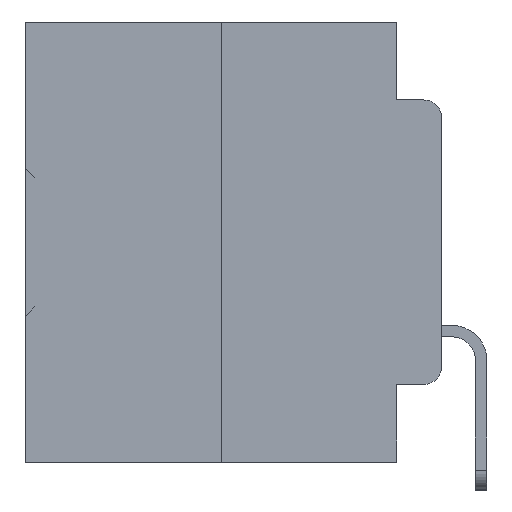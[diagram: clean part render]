
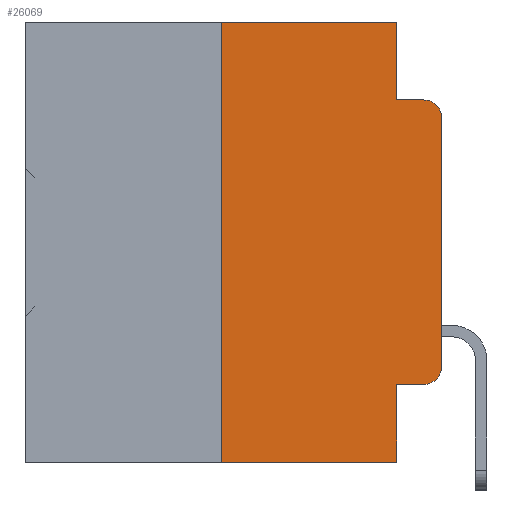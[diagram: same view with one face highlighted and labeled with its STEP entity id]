
A CAD part, left-side view. The second image highlights one B-rep face of the part: STEP entity #26069.
In plain terms, the highlighted planar face has unit normal (-1, 0, 0).
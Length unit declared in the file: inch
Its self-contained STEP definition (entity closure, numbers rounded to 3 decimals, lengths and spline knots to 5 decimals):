
#166 = LINE ( 'NONE', #28199, #23881 ) ;
#250 = VECTOR ( 'NONE', #28314, 39.37008 ) ;
#1336 = DIRECTION ( 'NONE',  ( -1., 0., 0. ) ) ;
#1528 = VERTEX_POINT ( 'NONE', #11129 ) ;
#2010 = VERTEX_POINT ( 'NONE', #10400 ) ;
#2981 = EDGE_CURVE ( 'NONE', #5622, #13626, #22046, .T. ) ;
#3457 = ORIENTED_EDGE ( 'NONE', *, *, #6452, .T. ) ;
#3941 = LINE ( 'NONE', #6048, #19441 ) ;
#4427 = CARTESIAN_POINT ( 'NONE',  ( 0., 0.473, 0. ) ) ;
#5622 = VERTEX_POINT ( 'NONE', #19685 ) ;
#5804 = DIRECTION ( 'NONE',  ( 0., -1., 0. ) ) ;
#6048 = CARTESIAN_POINT ( 'NONE',  ( 0., 0.051, 0. ) ) ;
#6452 = EDGE_CURVE ( 'NONE', #16078, #2010, #38901, .T. ) ;
#6487 = VERTEX_POINT ( 'NONE', #11929 ) ;
#6811 = VECTOR ( 'NONE', #35117, 39.37008 ) ;
#7681 = DIRECTION ( 'NONE',  ( 0., 0., 1. ) ) ;
#8719 = VECTOR ( 'NONE', #15376, 39.37008 ) ;
#9222 = DIRECTION ( 'NONE',  ( 0., 0., -1. ) ) ;
#10400 = CARTESIAN_POINT ( 'NONE',  ( 0., 0.02, -0.0885 ) ) ;
#10667 = VECTOR ( 'NONE', #7681, 39.37008 ) ;
#10784 = PLANE ( 'NONE',  #23205 ) ;
#10856 = CARTESIAN_POINT ( 'NONE',  ( 0., 0., 0. ) ) ;
#11129 = CARTESIAN_POINT ( 'NONE',  ( 0., 0.25, -0.5 ) ) ;
#11929 = CARTESIAN_POINT ( 'NONE',  ( 0., 0.051, -0.5 ) ) ;
#12894 = DIRECTION ( 'NONE',  ( 0., 0., -1. ) ) ;
#13626 = VERTEX_POINT ( 'NONE', #14405 ) ;
#13813 = VERTEX_POINT ( 'NONE', #39015 ) ;
#14405 = CARTESIAN_POINT ( 'NONE',  ( 0., 0.02, -0.4115 ) ) ;
#14736 = EDGE_CURVE ( 'NONE', #15678, #16078, #31298, .T. ) ;
#14965 = DIRECTION ( 'NONE',  ( -1., 0., 0. ) ) ;
#15132 = CARTESIAN_POINT ( 'NONE',  ( 0., 0.051, -0.4115 ) ) ;
#15240 = CARTESIAN_POINT ( 'NONE',  ( 0., 0.473, -0.5 ) ) ;
#15376 = DIRECTION ( 'NONE',  ( 0., -1., 0. ) ) ;
#15678 = VERTEX_POINT ( 'NONE', #32899 ) ;
#16078 = VERTEX_POINT ( 'NONE', #31957 ) ;
#17566 = EDGE_CURVE ( 'NONE', #5622, #6487, #3941, .T. ) ;
#17858 = LINE ( 'NONE', #15240, #8719 ) ;
#18710 = AXIS2_PLACEMENT_3D ( 'NONE', #19939, #1336, #22951 ) ;
#19043 = CARTESIAN_POINT ( 'NONE',  ( 0., 0.051, 0. ) ) ;
#19441 = VECTOR ( 'NONE', #9222, 39.37008 ) ;
#19590 = EDGE_CURVE ( 'NONE', #1528, #30109, #32742, .T. ) ;
#19685 = CARTESIAN_POINT ( 'NONE',  ( 0., 0.051, -0.4115 ) ) ;
#19939 = CARTESIAN_POINT ( 'NONE',  ( 0., 0.02, -0.3915 ) ) ;
#19947 = ORIENTED_EDGE ( 'NONE', *, *, #19590, .F. ) ;
#19952 = DIRECTION ( 'NONE',  ( 0., 0., -1. ) ) ;
#20078 = FACE_OUTER_BOUND ( 'NONE', #23715, .T. ) ;
#20436 = CARTESIAN_POINT ( 'NONE',  ( 0., 0.051, -0.0885 ) ) ;
#21294 = CARTESIAN_POINT ( 'NONE',  ( 0., 0.25, 0. ) ) ;
#22046 = LINE ( 'NONE', #15132, #37760 ) ;
#22318 = ORIENTED_EDGE ( 'NONE', *, *, #38192, .T. ) ;
#22951 = DIRECTION ( 'NONE',  ( 0., 0., -1. ) ) ;
#23205 = AXIS2_PLACEMENT_3D ( 'NONE', #4427, #37682, #19952 ) ;
#23630 = EDGE_CURVE ( 'NONE', #13813, #34739, #28907, .T. ) ;
#23715 = EDGE_LOOP ( 'NONE', ( #32924, #3457, #29691, #32461, #30164, #19947, #37547, #23726, #27433, #22318 ) ) ;
#23726 = ORIENTED_EDGE ( 'NONE', *, *, #17566, .F. ) ;
#23881 = VECTOR ( 'NONE', #31153, 39.37008 ) ;
#24675 = EDGE_CURVE ( 'NONE', #1528, #6487, #17858, .T. ) ;
#25370 = CARTESIAN_POINT ( 'NONE',  ( 0., 0.25, 0. ) ) ;
#26069 = ADVANCED_FACE ( 'NONE', ( #20078 ), #10784, .F. ) ;
#26359 = CARTESIAN_POINT ( 'NONE',  ( 0., 0.051, -0.0885 ) ) ;
#27433 = ORIENTED_EDGE ( 'NONE', *, *, #2981, .T. ) ;
#27586 = EDGE_CURVE ( 'NONE', #34739, #2010, #30940, .T. ) ;
#28199 = CARTESIAN_POINT ( 'NONE',  ( 0., 0.473, 0. ) ) ;
#28314 = DIRECTION ( 'NONE',  ( 0., 0., 1. ) ) ;
#28907 = LINE ( 'NONE', #19043, #35841 ) ;
#29691 = ORIENTED_EDGE ( 'NONE', *, *, #27586, .F. ) ;
#30109 = VERTEX_POINT ( 'NONE', #21294 ) ;
#30164 = ORIENTED_EDGE ( 'NONE', *, *, #37501, .F. ) ;
#30940 = LINE ( 'NONE', #26359, #6811 ) ;
#31153 = DIRECTION ( 'NONE',  ( 0., -1., 0. ) ) ;
#31298 = LINE ( 'NONE', #10856, #10667 ) ;
#31957 = CARTESIAN_POINT ( 'NONE',  ( 0., 0., -0.1085 ) ) ;
#32461 = ORIENTED_EDGE ( 'NONE', *, *, #23630, .F. ) ;
#32742 = LINE ( 'NONE', #25370, #250 ) ;
#32884 = CARTESIAN_POINT ( 'NONE',  ( 0., 0.02, -0.1085 ) ) ;
#32899 = CARTESIAN_POINT ( 'NONE',  ( 0., 0., -0.3915 ) ) ;
#32924 = ORIENTED_EDGE ( 'NONE', *, *, #14736, .T. ) ;
#34156 = AXIS2_PLACEMENT_3D ( 'NONE', #32884, #14965, #35835 ) ;
#34739 = VERTEX_POINT ( 'NONE', #20436 ) ;
#35117 = DIRECTION ( 'NONE',  ( 0., -1., 0. ) ) ;
#35835 = DIRECTION ( 'NONE',  ( 0., 0., -1. ) ) ;
#35841 = VECTOR ( 'NONE', #12894, 39.37008 ) ;
#37182 = CIRCLE ( 'NONE', #18710, 0.02 ) ;
#37501 = EDGE_CURVE ( 'NONE', #30109, #13813, #166, .T. ) ;
#37547 = ORIENTED_EDGE ( 'NONE', *, *, #24675, .T. ) ;
#37682 = DIRECTION ( 'NONE',  ( 1., 0., 0. ) ) ;
#37760 = VECTOR ( 'NONE', #5804, 39.37008 ) ;
#38192 = EDGE_CURVE ( 'NONE', #13626, #15678, #37182, .T. ) ;
#38901 = CIRCLE ( 'NONE', #34156, 0.02 ) ;
#39015 = CARTESIAN_POINT ( 'NONE',  ( 0., 0.051, 0. ) ) ;
